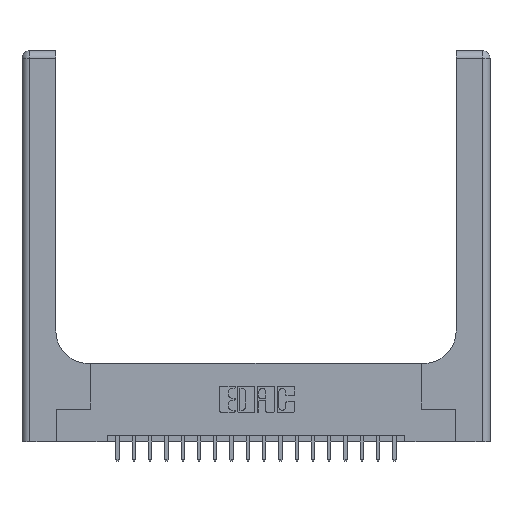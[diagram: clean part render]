
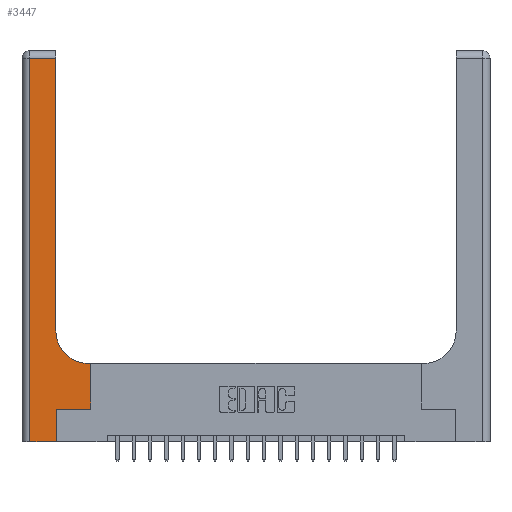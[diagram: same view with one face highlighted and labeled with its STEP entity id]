
A CAD part, top view. The second image highlights one B-rep face of the part: STEP entity #3447.
In plain terms, the highlighted planar face has unit normal (0, 0, 1).
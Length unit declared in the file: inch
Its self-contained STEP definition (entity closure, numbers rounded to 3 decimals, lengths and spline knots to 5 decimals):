
#200 = EDGE_CURVE ( 'NONE', #17034, #5719, #1913, .T. ) ;
#739 = LINE ( 'NONE', #11321, #10743 ) ;
#877 = CARTESIAN_POINT ( 'NONE',  ( 0.06, 2.94, 0.37 ) ) ;
#1392 = DIRECTION ( 'NONE',  ( -1., 0., 0. ) ) ;
#1621 = VERTEX_POINT ( 'NONE', #5036 ) ;
#1637 = EDGE_CURVE ( 'NONE', #15565, #1666, #10385, .T. ) ;
#1666 = VERTEX_POINT ( 'NONE', #16721 ) ;
#1870 = ORIENTED_EDGE ( 'NONE', *, *, #14767, .T. ) ;
#1907 = CARTESIAN_POINT ( 'NONE',  ( 0.528, 0.25, 0.37 ) ) ;
#1913 = LINE ( 'NONE', #7443, #10928 ) ;
#2561 = DIRECTION ( 'NONE',  ( -1., 0., 0. ) ) ;
#3021 = VECTOR ( 'NONE', #11942, 39.37008 ) ;
#3028 = DIRECTION ( 'NONE',  ( 0., -1., 0. ) ) ;
#3058 = EDGE_CURVE ( 'NONE', #8424, #17034, #7140, .T. ) ;
#3122 = EDGE_CURVE ( 'NONE', #1621, #11808, #12482, .T. ) ;
#3447 = ADVANCED_FACE ( 'NONE', ( #6146 ), #8708, .F. ) ;
#4030 = DIRECTION ( 'NONE',  ( -1., 0., 0. ) ) ;
#4266 = VECTOR ( 'NONE', #13386, 39.37008 ) ;
#4874 = LINE ( 'NONE', #7213, #10497 ) ;
#5036 = CARTESIAN_POINT ( 'NONE',  ( 0.51, 0.6, 0.37 ) ) ;
#5275 = ORIENTED_EDGE ( 'NONE', *, *, #3058, .T. ) ;
#5427 = DIRECTION ( 'NONE',  ( 0., 0., -1. ) ) ;
#5487 = VECTOR ( 'NONE', #1392, 39.37008 ) ;
#5607 = EDGE_CURVE ( 'NONE', #11398, #8595, #739, .T. ) ;
#5719 = VERTEX_POINT ( 'NONE', #19113 ) ;
#5767 = CARTESIAN_POINT ( 'NONE',  ( 0.265, 0.25, 0.37 ) ) ;
#6146 = FACE_OUTER_BOUND ( 'NONE', #11301, .T. ) ;
#6294 = LINE ( 'NONE', #12770, #8983 ) ;
#7140 = LINE ( 'NONE', #14003, #3021 ) ;
#7213 = CARTESIAN_POINT ( 'NONE',  ( 0.26, 3., 0.37 ) ) ;
#7443 = CARTESIAN_POINT ( 'NONE',  ( 0.265, 0., 0.37 ) ) ;
#8424 = VERTEX_POINT ( 'NONE', #14500 ) ;
#8595 = VERTEX_POINT ( 'NONE', #877 ) ;
#8708 = PLANE ( 'NONE',  #17797 ) ;
#8983 = VECTOR ( 'NONE', #3028, 39.37008 ) ;
#9195 = ORIENTED_EDGE ( 'NONE', *, *, #200, .T. ) ;
#9614 = CARTESIAN_POINT ( 'NONE',  ( 0.51, 0.85, 0.37 ) ) ;
#10005 = ORIENTED_EDGE ( 'NONE', *, *, #13508, .T. ) ;
#10385 = LINE ( 'NONE', #10618, #17439 ) ;
#10497 = VECTOR ( 'NONE', #14706, 39.37008 ) ;
#10618 = CARTESIAN_POINT ( 'NONE',  ( 0.528, 0.25, 0.37 ) ) ;
#10743 = VECTOR ( 'NONE', #4030, 39.37008 ) ;
#10928 = VECTOR ( 'NONE', #13915, 39.37008 ) ;
#11091 = LINE ( 'NONE', #15278, #5487 ) ;
#11163 = AXIS2_PLACEMENT_3D ( 'NONE', #9614, #11214, #12771 ) ;
#11187 = EDGE_CURVE ( 'NONE', #5719, #15565, #18156, .T. ) ;
#11214 = DIRECTION ( 'NONE',  ( 0., 0., -1. ) ) ;
#11301 = EDGE_LOOP ( 'NONE', ( #10005, #14208, #1870, #5275, #9195, #16238, #18196, #11370, #19688 ) ) ;
#11321 = CARTESIAN_POINT ( 'NONE',  ( 0., 2.94, 0.37 ) ) ;
#11370 = ORIENTED_EDGE ( 'NONE', *, *, #11418, .T. ) ;
#11398 = VERTEX_POINT ( 'NONE', #13648 ) ;
#11418 = EDGE_CURVE ( 'NONE', #1666, #1621, #11091, .T. ) ;
#11808 = VERTEX_POINT ( 'NONE', #19673 ) ;
#11942 = DIRECTION ( 'NONE',  ( 1., 0., 0. ) ) ;
#12482 = CIRCLE ( 'NONE', #11163, 0.25 ) ;
#12770 = CARTESIAN_POINT ( 'NONE',  ( 0.06, 3., 0.37 ) ) ;
#12771 = DIRECTION ( 'NONE',  ( 1., 0., 0. ) ) ;
#13212 = CARTESIAN_POINT ( 'NONE',  ( 0.265, 0., 0.37 ) ) ;
#13315 = CARTESIAN_POINT ( 'NONE',  ( 0., 3., 0.37 ) ) ;
#13386 = DIRECTION ( 'NONE',  ( 1., 0., 0. ) ) ;
#13508 = EDGE_CURVE ( 'NONE', #11808, #11398, #4874, .T. ) ;
#13648 = CARTESIAN_POINT ( 'NONE',  ( 0.26, 2.94, 0.37 ) ) ;
#13730 = DIRECTION ( 'NONE',  ( 0., 1., 0. ) ) ;
#13915 = DIRECTION ( 'NONE',  ( 0., 1., 0. ) ) ;
#14003 = CARTESIAN_POINT ( 'NONE',  ( 0., 0., 0.37 ) ) ;
#14208 = ORIENTED_EDGE ( 'NONE', *, *, #5607, .T. ) ;
#14500 = CARTESIAN_POINT ( 'NONE',  ( 0.06, 0., 0.37 ) ) ;
#14706 = DIRECTION ( 'NONE',  ( 0., 1., 0. ) ) ;
#14767 = EDGE_CURVE ( 'NONE', #8595, #8424, #6294, .T. ) ;
#15278 = CARTESIAN_POINT ( 'NONE',  ( 0.26, 0.6, 0.37 ) ) ;
#15565 = VERTEX_POINT ( 'NONE', #1907 ) ;
#16238 = ORIENTED_EDGE ( 'NONE', *, *, #11187, .T. ) ;
#16721 = CARTESIAN_POINT ( 'NONE',  ( 0.528, 0.6, 0.37 ) ) ;
#17034 = VERTEX_POINT ( 'NONE', #13212 ) ;
#17439 = VECTOR ( 'NONE', #13730, 39.37008 ) ;
#17797 = AXIS2_PLACEMENT_3D ( 'NONE', #13315, #5427, #2561 ) ;
#18156 = LINE ( 'NONE', #5767, #4266 ) ;
#18196 = ORIENTED_EDGE ( 'NONE', *, *, #1637, .T. ) ;
#19113 = CARTESIAN_POINT ( 'NONE',  ( 0.265, 0.25, 0.37 ) ) ;
#19673 = CARTESIAN_POINT ( 'NONE',  ( 0.26, 0.85, 0.37 ) ) ;
#19688 = ORIENTED_EDGE ( 'NONE', *, *, #3122, .T. ) ;
